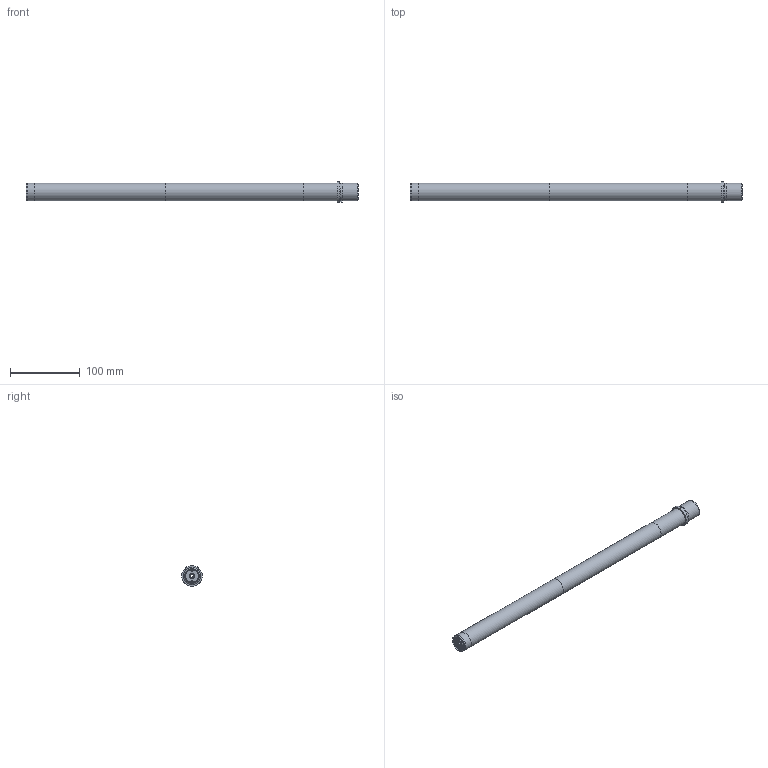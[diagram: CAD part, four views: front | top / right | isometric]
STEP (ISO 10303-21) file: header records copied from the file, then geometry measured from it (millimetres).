
FILE_DESCRIPTION(/* description */ (''),/* implementation_level */ '2;1');
FILE_NAME(/* name */ 'Tubee-22 Barrel.step',/* time_stamp */ '2021-04-26T16:11:08-04:00',/* author */ (''),/* organization */ (''),/* preprocessor_version */ 'ST-DEVELOPER v18.1',/* originating_system */ 'Autodesk Translation Framework v10.6.0.1341',/* authorisation */ '');
FILE_SCHEMA (('AUTOMOTIVE_DESIGN { 1 0 10303 214 3 1 1 }'));
Length unit declared in the file: inch
Products named in the file (2): AR22 Lined Barrel; Barrel, 16"
Assembly tree (1 placements, depth 2):
  AR22 Lined Barrel
    Barrel, 16"
Bounding box: 477.36 x 29.84 x 29.86 mm (x, y, z)
Volume: 215153.3 mm3; surface area: 75273.7 mm2
Topology: 5 solids, 5 shells, 227 faces, 580 edges, 372 vertices
Faces by surface type: bspline 134, cylinder 57, plane 26, cone 5, torus 5
Full cylindrical faces by diameter (mm): 3.2 x8, 5.753 x1, 8 x1, 8.3 x3, 19.101 x7, 20.637 x7, 21.291 x1, 24.905 x4, 25.222 x1, 25.367 x1, 29.845 x1
Entity records: 20853 total; most frequent: CARTESIAN_POINT 16201, ORIENTED_EDGE 1160, DIRECTION 645, EDGE_CURVE 580, VERTEX_POINT 372, B_SPLINE_CURVE_WITH_KNOTS 255, AXIS2_PLACEMENT_3D 250, EDGE_LOOP 246
